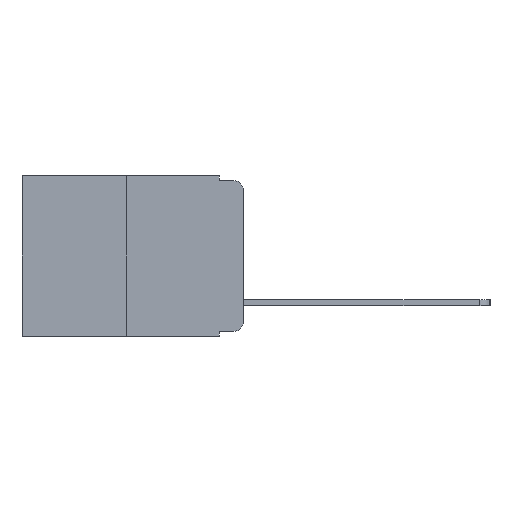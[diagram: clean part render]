
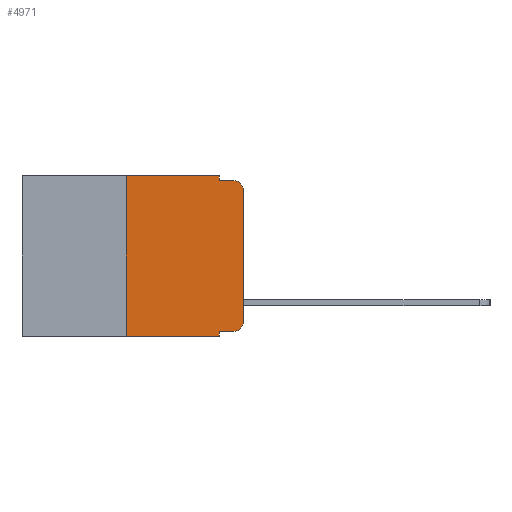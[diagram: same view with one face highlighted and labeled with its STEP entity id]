
A CAD part, left-side view. The second image highlights one B-rep face of the part: STEP entity #4971.
In plain terms, the highlighted planar face has unit normal (-1, 0, 0).
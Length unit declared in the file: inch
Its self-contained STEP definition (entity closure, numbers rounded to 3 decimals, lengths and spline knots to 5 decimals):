
#63 = ORIENTED_EDGE ( 'NONE', *, *, #1118, .F. ) ;
#354 = CARTESIAN_POINT ( 'NONE',  ( 0., 0.051, -0.333 ) ) ;
#370 = VERTEX_POINT ( 'NONE', #2076 ) ;
#505 = ORIENTED_EDGE ( 'NONE', *, *, #1807, .F. ) ;
#605 = ORIENTED_EDGE ( 'NONE', *, *, #5449, .F. ) ;
#607 = CARTESIAN_POINT ( 'NONE',  ( 0., 0.02, -0.03 ) ) ;
#717 = CARTESIAN_POINT ( 'NONE',  ( 0., 0.473, -0.343 ) ) ;
#773 = VECTOR ( 'NONE', #9494, 39.37008 ) ;
#850 = VECTOR ( 'NONE', #6802, 39.37008 ) ;
#877 = CARTESIAN_POINT ( 'NONE',  ( 0., 0.02, -0.01 ) ) ;
#949 = ORIENTED_EDGE ( 'NONE', *, *, #4259, .F. ) ;
#1057 = DIRECTION ( 'NONE',  ( 0., 0., -1. ) ) ;
#1118 = EDGE_CURVE ( 'NONE', #370, #3838, #5630, .T. ) ;
#1249 = ORIENTED_EDGE ( 'NONE', *, *, #10218, .T. ) ;
#1328 = DIRECTION ( 'NONE',  ( 0., -1., 0. ) ) ;
#1437 = CARTESIAN_POINT ( 'NONE',  ( 0., 0.25, 0. ) ) ;
#1501 = ORIENTED_EDGE ( 'NONE', *, *, #4792, .F. ) ;
#1672 = DIRECTION ( 'NONE',  ( 0., 0., -1. ) ) ;
#1684 = VECTOR ( 'NONE', #8371, 39.37008 ) ;
#1762 = DIRECTION ( 'NONE',  ( 0., -1., 0. ) ) ;
#1807 = EDGE_CURVE ( 'NONE', #3972, #370, #5750, .T. ) ;
#2058 = ORIENTED_EDGE ( 'NONE', *, *, #5384, .T. ) ;
#2076 = CARTESIAN_POINT ( 'NONE',  ( 0., 0.051, -0.01 ) ) ;
#2279 = VERTEX_POINT ( 'NONE', #10870 ) ;
#2352 = ORIENTED_EDGE ( 'NONE', *, *, #6509, .T. ) ;
#2483 = CARTESIAN_POINT ( 'NONE',  ( 0., 0.473, 0. ) ) ;
#2521 = AXIS2_PLACEMENT_3D ( 'NONE', #10150, #2639, #8616 ) ;
#2547 = AXIS2_PLACEMENT_3D ( 'NONE', #9173, #4197, #9986 ) ;
#2639 = DIRECTION ( 'NONE',  ( 1., 0., 0. ) ) ;
#2703 = ORIENTED_EDGE ( 'NONE', *, *, #11083, .T. ) ;
#2898 = CARTESIAN_POINT ( 'NONE',  ( 0., 0., -0.03 ) ) ;
#3172 = CARTESIAN_POINT ( 'NONE',  ( 0., 0.051, -0.343 ) ) ;
#3229 = VECTOR ( 'NONE', #7105, 39.37008 ) ;
#3548 = VECTOR ( 'NONE', #1057, 39.37008 ) ;
#3598 = CIRCLE ( 'NONE', #6117, 0.02 ) ;
#3629 = ORIENTED_EDGE ( 'NONE', *, *, #10532, .T. ) ;
#3763 = LINE ( 'NONE', #2483, #850 ) ;
#3838 = VERTEX_POINT ( 'NONE', #877 ) ;
#3923 = VERTEX_POINT ( 'NONE', #6998 ) ;
#3972 = VERTEX_POINT ( 'NONE', #4836 ) ;
#4073 = CARTESIAN_POINT ( 'NONE',  ( 0., 0.25, 0. ) ) ;
#4197 = DIRECTION ( 'NONE',  ( -1., 0., 0. ) ) ;
#4259 = EDGE_CURVE ( 'NONE', #2279, #8598, #5471, .T. ) ;
#4373 = PLANE ( 'NONE',  #2521 ) ;
#4377 = VECTOR ( 'NONE', #7081, 39.37008 ) ;
#4388 = VECTOR ( 'NONE', #1762, 39.37008 ) ;
#4526 = FACE_OUTER_BOUND ( 'NONE', #7952, .T. ) ;
#4747 = CIRCLE ( 'NONE', #2547, 0.02 ) ;
#4792 = EDGE_CURVE ( 'NONE', #9343, #5773, #10705, .T. ) ;
#4836 = CARTESIAN_POINT ( 'NONE',  ( 0., 0.051, 0. ) ) ;
#4971 = ADVANCED_FACE ( 'NONE', ( #4526 ), #4373, .F. ) ;
#5384 = EDGE_CURVE ( 'NONE', #9343, #9217, #8950, .T. ) ;
#5449 = EDGE_CURVE ( 'NONE', #8598, #3972, #3763, .T. ) ;
#5471 = LINE ( 'NONE', #1437, #3229 ) ;
#5630 = LINE ( 'NONE', #8045, #773 ) ;
#5750 = LINE ( 'NONE', #10766, #3548 ) ;
#5773 = VERTEX_POINT ( 'NONE', #3172 ) ;
#6117 = AXIS2_PLACEMENT_3D ( 'NONE', #607, #6948, #1672 ) ;
#6192 = CARTESIAN_POINT ( 'NONE',  ( 0., 0., 0. ) ) ;
#6486 = VECTOR ( 'NONE', #1328, 39.37008 ) ;
#6509 = EDGE_CURVE ( 'NONE', #9217, #3923, #4747, .T. ) ;
#6802 = DIRECTION ( 'NONE',  ( 0., -1., 0. ) ) ;
#6884 = VERTEX_POINT ( 'NONE', #2898 ) ;
#6948 = DIRECTION ( 'NONE',  ( -1., 0., 0. ) ) ;
#6998 = CARTESIAN_POINT ( 'NONE',  ( 0., 0., -0.313 ) ) ;
#7081 = DIRECTION ( 'NONE',  ( 0., 0., 1. ) ) ;
#7105 = DIRECTION ( 'NONE',  ( 0., 0., 1. ) ) ;
#7382 = CARTESIAN_POINT ( 'NONE',  ( 0., 0.02, -0.333 ) ) ;
#7539 = CARTESIAN_POINT ( 'NONE',  ( 0., 0.051, 0. ) ) ;
#7952 = EDGE_LOOP ( 'NONE', ( #3629, #2703, #63, #505, #605, #949, #1249, #1501, #2058, #2352 ) ) ;
#8045 = CARTESIAN_POINT ( 'NONE',  ( 0., 0.051, -0.01 ) ) ;
#8371 = DIRECTION ( 'NONE',  ( 0., 0., -1. ) ) ;
#8598 = VERTEX_POINT ( 'NONE', #4073 ) ;
#8616 = DIRECTION ( 'NONE',  ( 0., 0., -1. ) ) ;
#8837 = LINE ( 'NONE', #6192, #4377 ) ;
#8950 = LINE ( 'NONE', #10767, #6486 ) ;
#9173 = CARTESIAN_POINT ( 'NONE',  ( 0., 0.02, -0.313 ) ) ;
#9217 = VERTEX_POINT ( 'NONE', #7382 ) ;
#9343 = VERTEX_POINT ( 'NONE', #354 ) ;
#9494 = DIRECTION ( 'NONE',  ( 0., -1., 0. ) ) ;
#9986 = DIRECTION ( 'NONE',  ( 0., 0., -1. ) ) ;
#10150 = CARTESIAN_POINT ( 'NONE',  ( 0., 0.473, 0. ) ) ;
#10218 = EDGE_CURVE ( 'NONE', #2279, #5773, #10955, .T. ) ;
#10532 = EDGE_CURVE ( 'NONE', #3923, #6884, #8837, .T. ) ;
#10705 = LINE ( 'NONE', #7539, #1684 ) ;
#10766 = CARTESIAN_POINT ( 'NONE',  ( 0., 0.051, 0. ) ) ;
#10767 = CARTESIAN_POINT ( 'NONE',  ( 0., 0.051, -0.333 ) ) ;
#10870 = CARTESIAN_POINT ( 'NONE',  ( 0., 0.25, -0.343 ) ) ;
#10955 = LINE ( 'NONE', #717, #4388 ) ;
#11083 = EDGE_CURVE ( 'NONE', #6884, #3838, #3598, .T. ) ;
